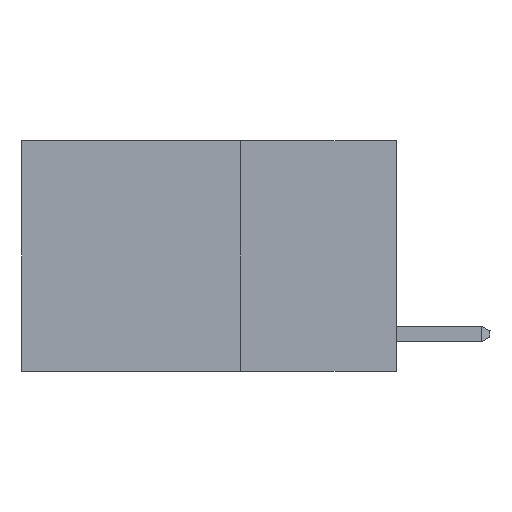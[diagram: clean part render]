
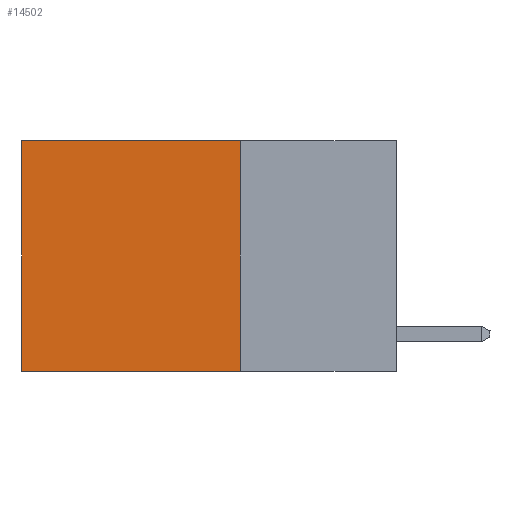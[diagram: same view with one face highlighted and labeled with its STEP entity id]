
A CAD part, left-side view. The second image highlights one B-rep face of the part: STEP entity #14502.
In plain terms, the highlighted planar face has unit normal (-1, 0, 0).
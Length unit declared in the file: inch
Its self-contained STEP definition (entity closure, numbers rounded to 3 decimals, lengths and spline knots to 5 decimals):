
#182 = PLANE ( 'NONE',  #2145 ) ;
#725 = ORIENTED_EDGE ( 'NONE', *, *, #13286, .T. ) ;
#806 = DIRECTION ( 'NONE',  ( 0., 1., 0. ) ) ;
#1624 = VECTOR ( 'NONE', #806, 39.37008 ) ;
#2145 = AXIS2_PLACEMENT_3D ( 'NONE', #4899, #6353, #18003 ) ;
#2178 = CARTESIAN_POINT ( 'NONE',  ( 0.2625, 0.6, 0. ) ) ;
#2198 = EDGE_CURVE ( 'NONE', #16960, #8232, #7012, .T. ) ;
#2729 = CARTESIAN_POINT ( 'NONE',  ( 0.2625, 0.6, -0.37 ) ) ;
#3047 = DIRECTION ( 'NONE',  ( 0., 0., -1. ) ) ;
#3176 = CARTESIAN_POINT ( 'NONE',  ( 0.2625, 0.25, 0. ) ) ;
#3880 = DIRECTION ( 'NONE',  ( 0., 1., 0. ) ) ;
#4716 = LINE ( 'NONE', #5196, #1624 ) ;
#4899 = CARTESIAN_POINT ( 'NONE',  ( 0.2625, 0.25, 0. ) ) ;
#5196 = CARTESIAN_POINT ( 'NONE',  ( 0.2625, 0.25, 0. ) ) ;
#5357 = DIRECTION ( 'NONE',  ( 0., 0., -1. ) ) ;
#6353 = DIRECTION ( 'NONE',  ( 1., 0., 0. ) ) ;
#6916 = CARTESIAN_POINT ( 'NONE',  ( 0.2625, 0.25, -0.37 ) ) ;
#7012 = LINE ( 'NONE', #17220, #17681 ) ;
#8232 = VERTEX_POINT ( 'NONE', #2729 ) ;
#9566 = EDGE_CURVE ( 'NONE', #18678, #16960, #17322, .T. ) ;
#10552 = EDGE_CURVE ( 'NONE', #18740, #8232, #16815, .T. ) ;
#12885 = CARTESIAN_POINT ( 'NONE',  ( 0.2625, 0.25, 0. ) ) ;
#13286 = EDGE_CURVE ( 'NONE', #18678, #18740, #4716, .T. ) ;
#14216 = CARTESIAN_POINT ( 'NONE',  ( 0.2625, 0.6, 0. ) ) ;
#14502 = ADVANCED_FACE ( 'NONE', ( #17368 ), #182, .F. ) ;
#15661 = ORIENTED_EDGE ( 'NONE', *, *, #2198, .F. ) ;
#16170 = VECTOR ( 'NONE', #3047, 39.37008 ) ;
#16815 = LINE ( 'NONE', #14216, #18677 ) ;
#16960 = VERTEX_POINT ( 'NONE', #6916 ) ;
#17056 = EDGE_LOOP ( 'NONE', ( #18511, #15661, #18632, #725 ) ) ;
#17220 = CARTESIAN_POINT ( 'NONE',  ( 0.2625, 0.25, -0.37 ) ) ;
#17322 = LINE ( 'NONE', #3176, #16170 ) ;
#17368 = FACE_OUTER_BOUND ( 'NONE', #17056, .T. ) ;
#17681 = VECTOR ( 'NONE', #3880, 39.37008 ) ;
#18003 = DIRECTION ( 'NONE',  ( 0., 0., -1. ) ) ;
#18511 = ORIENTED_EDGE ( 'NONE', *, *, #10552, .T. ) ;
#18632 = ORIENTED_EDGE ( 'NONE', *, *, #9566, .F. ) ;
#18677 = VECTOR ( 'NONE', #5357, 39.37008 ) ;
#18678 = VERTEX_POINT ( 'NONE', #12885 ) ;
#18740 = VERTEX_POINT ( 'NONE', #2178 ) ;
